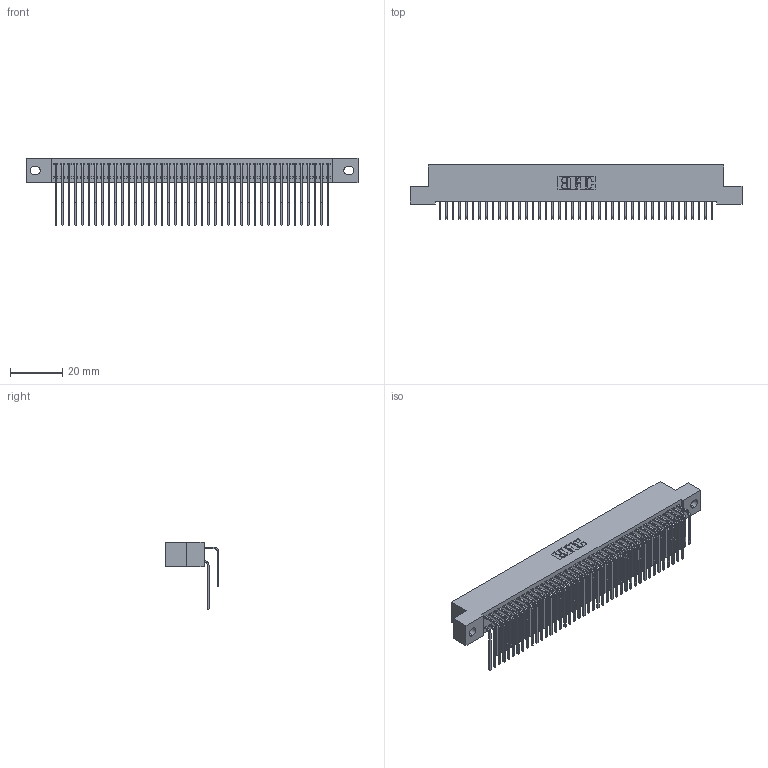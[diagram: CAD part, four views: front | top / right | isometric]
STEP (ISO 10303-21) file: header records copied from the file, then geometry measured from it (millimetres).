
FILE_DESCRIPTION (( 'STEP AP203' ), '1' );
FILE_NAME ('392-084-559-202.STEP', '2018-08-18T04:52:18', ( '' ), ( '' ), 'SwSTEP 2.0', 'SolidWorks 2016', '' );
FILE_SCHEMA (( 'CONFIG_CONTROL_DESIGN' ));
Length unit declared in the file: inch
Products named in the file (4): 345-292-001_559 Tail - 2; 392-084-559-202; 342 Part_.128 Slot; 345-292-001_558 559 Tail - 1
Assembly tree (85 placements, depth 2):
  392-084-559-202
    342 Part_.128 Slot
    345-292-001_558 559 Tail - 1  x42
    345-292-001_559 Tail - 2  x42
Bounding box: 127 x 20.64 x 25.78 mm (x, y, z)
Volume: 11843.4 mm3; surface area: 21229.6 mm2
Topology: 85 solids, 85 shells, 4650 faces, 13835 edges, 9110 vertices
Faces by surface type: plane 3262, cylinder 1388
Entity records: 28807 total; most frequent: CARTESIAN_POINT 4825, ORIENTED_EDGE 4710, DIRECTION 4103, EDGE_CURVE 2355, LINE 2187, VECTOR 2187, VERTEX_POINT 1566, AXIS2_PLACEMENT_3D 958
